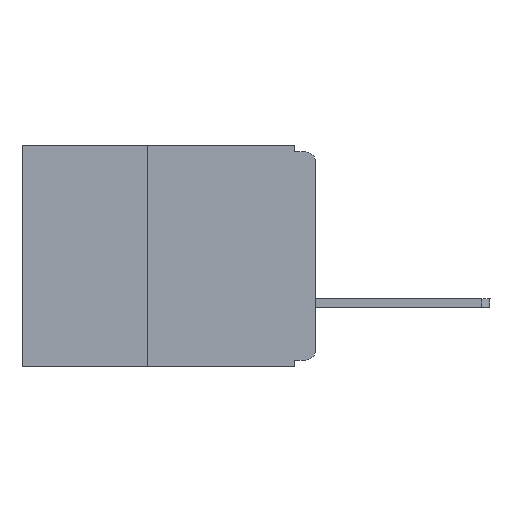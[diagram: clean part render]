
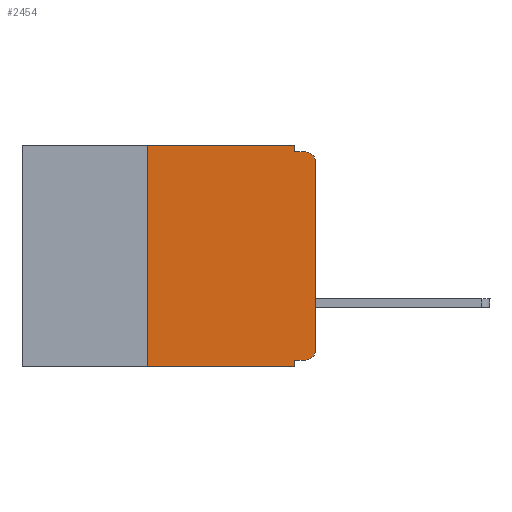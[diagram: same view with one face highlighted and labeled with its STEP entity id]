
A CAD part, left-side view. The second image highlights one B-rep face of the part: STEP entity #2454.
In plain terms, the highlighted planar face has unit normal (-1, 0, 0).
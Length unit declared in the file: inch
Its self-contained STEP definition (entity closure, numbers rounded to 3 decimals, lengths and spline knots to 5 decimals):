
#232 = CARTESIAN_POINT ( 'NONE',  ( 0., 0.437, -0.33 ) ) ;
#283 = CARTESIAN_POINT ( 'NONE',  ( 0., 0.25, -0.33 ) ) ;
#317 = LINE ( 'NONE', #232, #6496 ) ;
#690 = VERTEX_POINT ( 'NONE', #3725 ) ;
#753 = EDGE_CURVE ( 'NONE', #9614, #1846, #9459, .T. ) ;
#996 = DIRECTION ( 'NONE',  ( -1., 0., 0. ) ) ;
#1121 = PLANE ( 'NONE',  #3754 ) ;
#1161 = EDGE_CURVE ( 'NONE', #1846, #690, #11505, .T. ) ;
#1175 = DIRECTION ( 'NONE',  ( 0., -1., 0. ) ) ;
#1243 = CARTESIAN_POINT ( 'NONE',  ( 0., 0.437, 0. ) ) ;
#1317 = CARTESIAN_POINT ( 'NONE',  ( 0., 0.031, 0. ) ) ;
#1363 = EDGE_CURVE ( 'NONE', #11381, #9993, #7651, .T. ) ;
#1733 = VECTOR ( 'NONE', #5977, 39.37008 ) ;
#1846 = VERTEX_POINT ( 'NONE', #9323 ) ;
#1892 = DIRECTION ( 'NONE',  ( 0., -1., 0. ) ) ;
#2076 = ORIENTED_EDGE ( 'NONE', *, *, #1363, .F. ) ;
#2189 = DIRECTION ( 'NONE',  ( 0., 0., -1. ) ) ;
#2287 = CARTESIAN_POINT ( 'NONE',  ( 0., 0., 0. ) ) ;
#2454 = ADVANCED_FACE ( 'NONE', ( #2536 ), #1121, .F. ) ;
#2536 = FACE_OUTER_BOUND ( 'NONE', #11114, .T. ) ;
#2709 = EDGE_CURVE ( 'NONE', #3301, #9993, #317, .T. ) ;
#2798 = DIRECTION ( 'NONE',  ( 0., -1., 0. ) ) ;
#2891 = LINE ( 'NONE', #8989, #1733 ) ;
#2899 = CIRCLE ( 'NONE', #8102, 0.015 ) ;
#3054 = VECTOR ( 'NONE', #1892, 39.37008 ) ;
#3301 = VERTEX_POINT ( 'NONE', #283 ) ;
#3524 = DIRECTION ( 'NONE',  ( 0., 0., -1. ) ) ;
#3725 = CARTESIAN_POINT ( 'NONE',  ( 0., 0.031, -0.01 ) ) ;
#3736 = VERTEX_POINT ( 'NONE', #8364 ) ;
#3754 = AXIS2_PLACEMENT_3D ( 'NONE', #1243, #7735, #7866 ) ;
#3765 = VERTEX_POINT ( 'NONE', #10502 ) ;
#3822 = CARTESIAN_POINT ( 'NONE',  ( 0., 0.015, -0.025 ) ) ;
#3863 = ORIENTED_EDGE ( 'NONE', *, *, #10861, .T. ) ;
#4073 = CARTESIAN_POINT ( 'NONE',  ( 0., 0.015, -0.305 ) ) ;
#4267 = EDGE_CURVE ( 'NONE', #9888, #11381, #9587, .T. ) ;
#4547 = ORIENTED_EDGE ( 'NONE', *, *, #8902, .T. ) ;
#4714 = CARTESIAN_POINT ( 'NONE',  ( 0., 0.437, 0. ) ) ;
#4719 = CARTESIAN_POINT ( 'NONE',  ( 0., 0.031, -0.32 ) ) ;
#5185 = DIRECTION ( 'NONE',  ( 0., 0., 1. ) ) ;
#5250 = CARTESIAN_POINT ( 'NONE',  ( 0., 0.25, 0. ) ) ;
#5343 = VERTEX_POINT ( 'NONE', #8046 ) ;
#5382 = CARTESIAN_POINT ( 'NONE',  ( 0., 0.031, -0.33 ) ) ;
#5421 = VECTOR ( 'NONE', #2189, 39.37008 ) ;
#5679 = DIRECTION ( 'NONE',  ( 0., 1., 0. ) ) ;
#5977 = DIRECTION ( 'NONE',  ( 0., 0., 1. ) ) ;
#6288 = VECTOR ( 'NONE', #3524, 39.37008 ) ;
#6294 = LINE ( 'NONE', #2287, #6440 ) ;
#6440 = VECTOR ( 'NONE', #5185, 39.37008 ) ;
#6496 = VECTOR ( 'NONE', #1175, 39.37008 ) ;
#6759 = ORIENTED_EDGE ( 'NONE', *, *, #8908, .T. ) ;
#6991 = DIRECTION ( 'NONE',  ( 0., 0., -1. ) ) ;
#7651 = LINE ( 'NONE', #5382, #6288 ) ;
#7735 = DIRECTION ( 'NONE',  ( 1., 0., 0. ) ) ;
#7866 = DIRECTION ( 'NONE',  ( 0., 0., -1. ) ) ;
#7973 = ORIENTED_EDGE ( 'NONE', *, *, #753, .F. ) ;
#8023 = CARTESIAN_POINT ( 'NONE',  ( 0., 0.031, -0.33 ) ) ;
#8046 = CARTESIAN_POINT ( 'NONE',  ( 0., 0., -0.025 ) ) ;
#8102 = AXIS2_PLACEMENT_3D ( 'NONE', #4073, #9849, #6991 ) ;
#8364 = CARTESIAN_POINT ( 'NONE',  ( 0., 0.015, -0.01 ) ) ;
#8748 = ORIENTED_EDGE ( 'NONE', *, *, #10449, .F. ) ;
#8789 = CARTESIAN_POINT ( 'NONE',  ( 0., 0.015, -0.32 ) ) ;
#8902 = EDGE_CURVE ( 'NONE', #3765, #5343, #6294, .T. ) ;
#8908 = EDGE_CURVE ( 'NONE', #9888, #3765, #2899, .T. ) ;
#8989 = CARTESIAN_POINT ( 'NONE',  ( 0., 0.25, -0.33 ) ) ;
#9075 = LINE ( 'NONE', #11244, #10860 ) ;
#9323 = CARTESIAN_POINT ( 'NONE',  ( 0., 0.031, 0. ) ) ;
#9381 = AXIS2_PLACEMENT_3D ( 'NONE', #3822, #996, #9596 ) ;
#9459 = LINE ( 'NONE', #4714, #3054 ) ;
#9587 = LINE ( 'NONE', #11364, #10629 ) ;
#9596 = DIRECTION ( 'NONE',  ( 0., 0., -1. ) ) ;
#9614 = VERTEX_POINT ( 'NONE', #5250 ) ;
#9849 = DIRECTION ( 'NONE',  ( -1., 0., 0. ) ) ;
#9888 = VERTEX_POINT ( 'NONE', #8789 ) ;
#9979 = ORIENTED_EDGE ( 'NONE', *, *, #1161, .F. ) ;
#9993 = VERTEX_POINT ( 'NONE', #8023 ) ;
#10449 = EDGE_CURVE ( 'NONE', #3301, #9614, #2891, .T. ) ;
#10502 = CARTESIAN_POINT ( 'NONE',  ( 0., 0., -0.305 ) ) ;
#10629 = VECTOR ( 'NONE', #5679, 39.37008 ) ;
#10860 = VECTOR ( 'NONE', #2798, 39.37008 ) ;
#10861 = EDGE_CURVE ( 'NONE', #5343, #3736, #11181, .T. ) ;
#11114 = EDGE_LOOP ( 'NONE', ( #4547, #3863, #12235, #9979, #7973, #8748, #11345, #2076, #12219, #6759 ) ) ;
#11181 = CIRCLE ( 'NONE', #9381, 0.015 ) ;
#11244 = CARTESIAN_POINT ( 'NONE',  ( 0., 0., -0.01 ) ) ;
#11345 = ORIENTED_EDGE ( 'NONE', *, *, #2709, .T. ) ;
#11364 = CARTESIAN_POINT ( 'NONE',  ( 0., 0., -0.32 ) ) ;
#11381 = VERTEX_POINT ( 'NONE', #4719 ) ;
#11501 = EDGE_CURVE ( 'NONE', #690, #3736, #9075, .T. ) ;
#11505 = LINE ( 'NONE', #1317, #5421 ) ;
#12219 = ORIENTED_EDGE ( 'NONE', *, *, #4267, .F. ) ;
#12235 = ORIENTED_EDGE ( 'NONE', *, *, #11501, .F. ) ;
